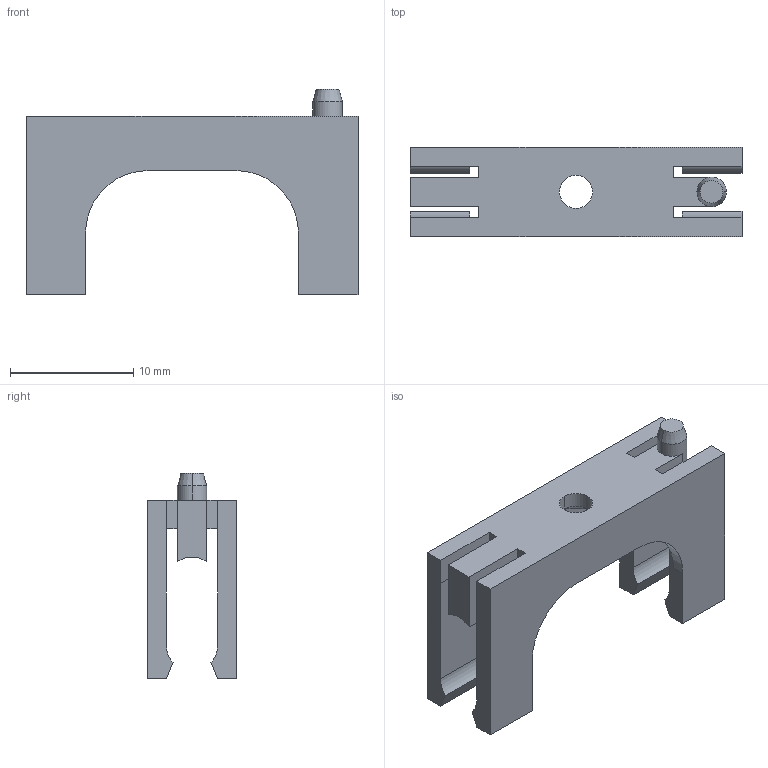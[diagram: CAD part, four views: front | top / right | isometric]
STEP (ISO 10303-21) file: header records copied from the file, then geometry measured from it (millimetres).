
FILE_DESCRIPTION (( 'STEP AP214' ), '1' );
FILE_NAME ('520-220-001.STEP', '2023-04-05T17:32:39', ( '' ), ( '' ), 'SwSTEP 2.0', 'SolidWorks 2020', '' );
FILE_SCHEMA (( 'AUTOMOTIVE_DESIGN' ));
Length unit declared in the file: inch
Products named in the file (1): 520-220-001
Bounding box: 26.92 x 7.24 x 16.69 mm (x, y, z)
Volume: 896.6 mm3; surface area: 1491.7 mm2
Topology: 1 solids, 1 shells, 64 faces, 180 edges, 118 vertices
Faces by surface type: plane 46, cylinder 16, cone 2
Entity records: 2109 total; most frequent: CARTESIAN_POINT 383, ORIENTED_EDGE 360, DIRECTION 341, EDGE_CURVE 180, LINE 145, VECTOR 145, VERTEX_POINT 118, AXIS2_PLACEMENT_3D 98
